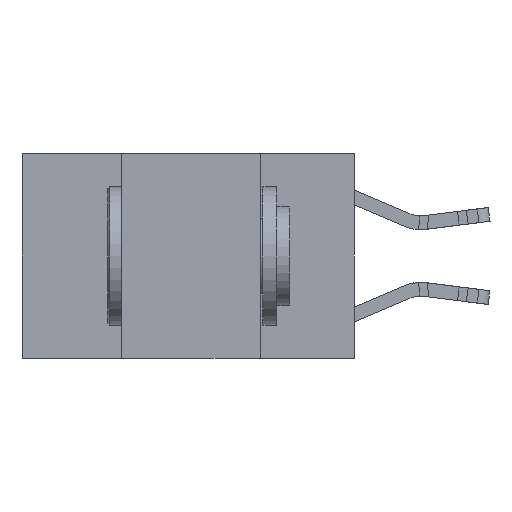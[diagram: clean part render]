
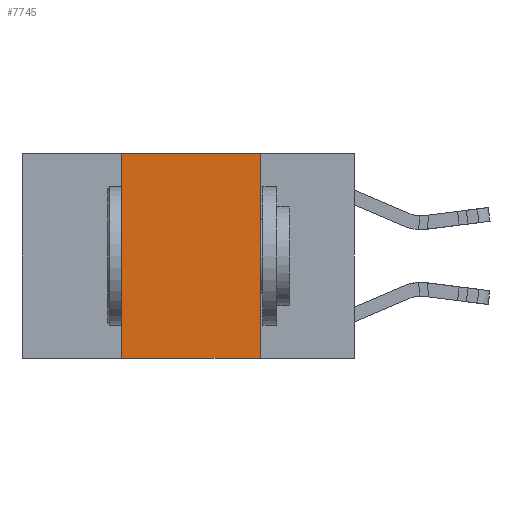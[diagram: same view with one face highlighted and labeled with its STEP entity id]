
A CAD part, left-side view. The second image highlights one B-rep face of the part: STEP entity #7745.
In plain terms, the highlighted planar face has unit normal (-1, 0, 0).
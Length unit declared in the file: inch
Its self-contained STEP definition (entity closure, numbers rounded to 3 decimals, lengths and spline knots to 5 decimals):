
#49 = VECTOR ( 'NONE', #15189, 39.37008 ) ;
#1592 = FACE_OUTER_BOUND ( 'NONE', #27347, .T. ) ;
#1750 = DIRECTION ( 'NONE',  ( 1., 0., 0. ) ) ;
#1801 = CARTESIAN_POINT ( 'NONE',  ( 0., 0.17, 0. ) ) ;
#2144 = VECTOR ( 'NONE', #20766, 39.37008 ) ;
#3827 = DIRECTION ( 'NONE',  ( 0., 0., -1. ) ) ;
#5119 = EDGE_CURVE ( 'NONE', #21830, #26493, #5805, .T. ) ;
#5805 = LINE ( 'NONE', #25759, #8064 ) ;
#5951 = DIRECTION ( 'NONE',  ( 0., 0., 1. ) ) ;
#7745 = ADVANCED_FACE ( 'NONE', ( #1592 ), #11344, .F. ) ;
#7835 = LINE ( 'NONE', #17608, #49 ) ;
#8064 = VECTOR ( 'NONE', #5951, 39.37008 ) ;
#10681 = CARTESIAN_POINT ( 'NONE',  ( 0., 0.17, 0. ) ) ;
#11344 = PLANE ( 'NONE',  #31174 ) ;
#13905 = EDGE_CURVE ( 'NONE', #26493, #29636, #7835, .T. ) ;
#15189 = DIRECTION ( 'NONE',  ( 0., -1., 0. ) ) ;
#15849 = DIRECTION ( 'NONE',  ( 0., -1., 0. ) ) ;
#16779 = VERTEX_POINT ( 'NONE', #24754 ) ;
#17608 = CARTESIAN_POINT ( 'NONE',  ( 0., 0.6, 0. ) ) ;
#20309 = VECTOR ( 'NONE', #15849, 39.37008 ) ;
#20353 = CARTESIAN_POINT ( 'NONE',  ( 0., 0.42, 0. ) ) ;
#20766 = DIRECTION ( 'NONE',  ( 0., 0., -1. ) ) ;
#20974 = CARTESIAN_POINT ( 'NONE',  ( 0., 0.6, -0.37 ) ) ;
#21830 = VERTEX_POINT ( 'NONE', #23072 ) ;
#23010 = LINE ( 'NONE', #10681, #2144 ) ;
#23072 = CARTESIAN_POINT ( 'NONE',  ( 0., 0.42, -0.37 ) ) ;
#23213 = LINE ( 'NONE', #20974, #20309 ) ;
#23491 = EDGE_CURVE ( 'NONE', #29636, #16779, #23010, .T. ) ;
#23657 = CARTESIAN_POINT ( 'NONE',  ( 0., 0.6, 0. ) ) ;
#24449 = ORIENTED_EDGE ( 'NONE', *, *, #5119, .F. ) ;
#24754 = CARTESIAN_POINT ( 'NONE',  ( 0., 0.17, -0.37 ) ) ;
#25759 = CARTESIAN_POINT ( 'NONE',  ( 0., 0.42, 0. ) ) ;
#26493 = VERTEX_POINT ( 'NONE', #20353 ) ;
#27117 = ORIENTED_EDGE ( 'NONE', *, *, #23491, .F. ) ;
#27347 = EDGE_LOOP ( 'NONE', ( #27117, #29552, #24449, #31409 ) ) ;
#29552 = ORIENTED_EDGE ( 'NONE', *, *, #13905, .F. ) ;
#29636 = VERTEX_POINT ( 'NONE', #1801 ) ;
#31174 = AXIS2_PLACEMENT_3D ( 'NONE', #23657, #1750, #3827 ) ;
#31409 = ORIENTED_EDGE ( 'NONE', *, *, #31486, .T. ) ;
#31486 = EDGE_CURVE ( 'NONE', #21830, #16779, #23213, .T. ) ;
